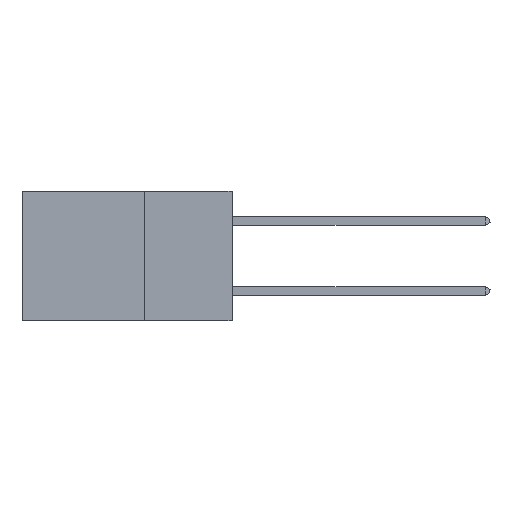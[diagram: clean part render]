
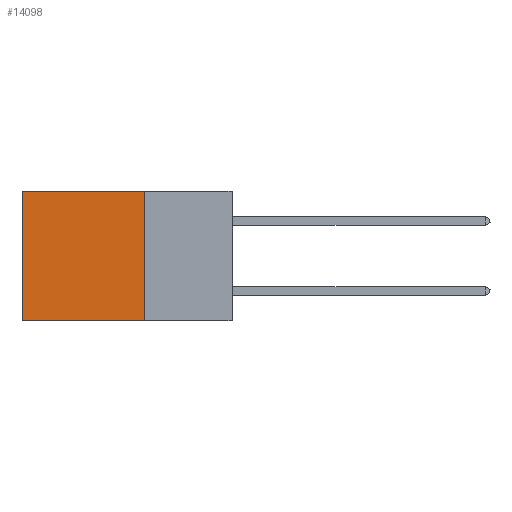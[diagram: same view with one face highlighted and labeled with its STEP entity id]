
A CAD part, left-side view. The second image highlights one B-rep face of the part: STEP entity #14098.
In plain terms, the highlighted planar face has unit normal (-1, 0, 0).
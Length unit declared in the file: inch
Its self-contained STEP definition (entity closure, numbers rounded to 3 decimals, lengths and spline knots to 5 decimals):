
#3184 = ORIENTED_EDGE ( 'NONE', *, *, #10750, .T. ) ;
#4280 = DIRECTION ( 'NONE',  ( 0., 0., -1. ) ) ;
#5220 = CARTESIAN_POINT ( 'NONE',  ( 0.2875, 0.25, 0. ) ) ;
#5475 = CARTESIAN_POINT ( 'NONE',  ( 0.2875, 0.6, 0. ) ) ;
#5669 = DIRECTION ( 'NONE',  ( 0., 1., 0. ) ) ;
#6836 = CARTESIAN_POINT ( 'NONE',  ( 0.2875, 0.25, -0.37 ) ) ;
#7341 = AXIS2_PLACEMENT_3D ( 'NONE', #20095, #23433, #4280 ) ;
#10750 = EDGE_CURVE ( 'NONE', #35800, #27158, #19478, .T. ) ;
#11232 = CARTESIAN_POINT ( 'NONE',  ( 0.2875, 0.25, 0. ) ) ;
#14098 = ADVANCED_FACE ( 'NONE', ( #14242 ), #20234, .F. ) ;
#14242 = FACE_OUTER_BOUND ( 'NONE', #36305, .T. ) ;
#14674 = LINE ( 'NONE', #33047, #39958 ) ;
#16408 = DIRECTION ( 'NONE',  ( 0., 1., 0. ) ) ;
#17288 = DIRECTION ( 'NONE',  ( 0., 0., -1. ) ) ;
#17602 = VERTEX_POINT ( 'NONE', #40854 ) ;
#17867 = CARTESIAN_POINT ( 'NONE',  ( 0.2875, 0.6, -0.37 ) ) ;
#19025 = EDGE_CURVE ( 'NONE', #17602, #36184, #28417, .T. ) ;
#19478 = LINE ( 'NONE', #31151, #27921 ) ;
#20095 = CARTESIAN_POINT ( 'NONE',  ( 0.2875, 0.25, 0. ) ) ;
#20234 = PLANE ( 'NONE',  #7341 ) ;
#22224 = VECTOR ( 'NONE', #24373, 39.37008 ) ;
#23218 = LINE ( 'NONE', #5220, #22224 ) ;
#23433 = DIRECTION ( 'NONE',  ( 1., 0., 0. ) ) ;
#24373 = DIRECTION ( 'NONE',  ( 0., 0., -1. ) ) ;
#26931 = EDGE_CURVE ( 'NONE', #27158, #36184, #14674, .T. ) ;
#27158 = VERTEX_POINT ( 'NONE', #5475 ) ;
#27433 = VECTOR ( 'NONE', #16408, 39.37008 ) ;
#27921 = VECTOR ( 'NONE', #5669, 39.37008 ) ;
#28417 = LINE ( 'NONE', #6836, #27433 ) ;
#29592 = ORIENTED_EDGE ( 'NONE', *, *, #36223, .F. ) ;
#31151 = CARTESIAN_POINT ( 'NONE',  ( 0.2875, 0.25, 0. ) ) ;
#33047 = CARTESIAN_POINT ( 'NONE',  ( 0.2875, 0.6, 0. ) ) ;
#35800 = VERTEX_POINT ( 'NONE', #11232 ) ;
#36184 = VERTEX_POINT ( 'NONE', #17867 ) ;
#36223 = EDGE_CURVE ( 'NONE', #35800, #17602, #23218, .T. ) ;
#36305 = EDGE_LOOP ( 'NONE', ( #40728, #36585, #29592, #3184 ) ) ;
#36585 = ORIENTED_EDGE ( 'NONE', *, *, #19025, .F. ) ;
#39958 = VECTOR ( 'NONE', #17288, 39.37008 ) ;
#40728 = ORIENTED_EDGE ( 'NONE', *, *, #26931, .T. ) ;
#40854 = CARTESIAN_POINT ( 'NONE',  ( 0.2875, 0.25, -0.37 ) ) ;
